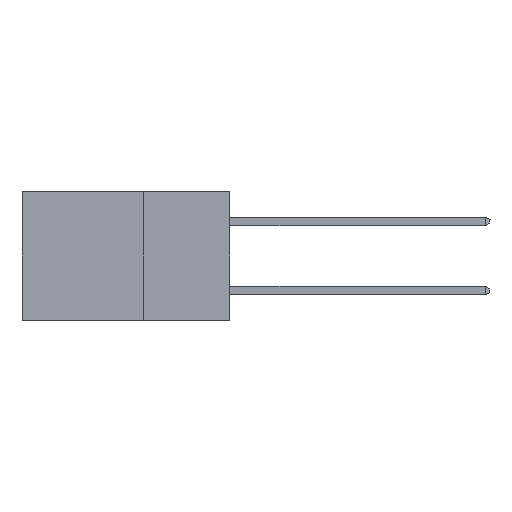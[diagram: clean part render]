
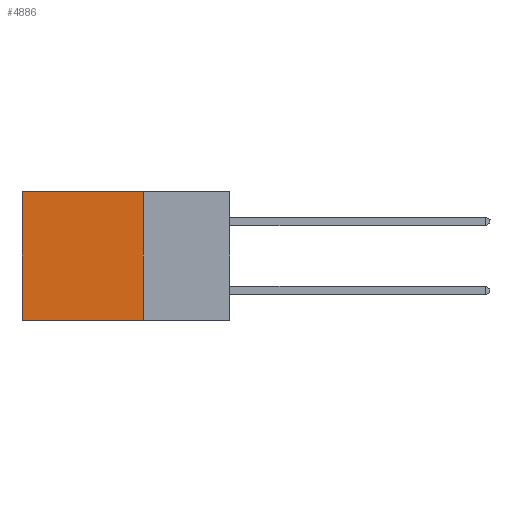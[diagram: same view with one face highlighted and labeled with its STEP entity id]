
A CAD part, left-side view. The second image highlights one B-rep face of the part: STEP entity #4886.
In plain terms, the highlighted planar face has unit normal (-1, 0, 0).
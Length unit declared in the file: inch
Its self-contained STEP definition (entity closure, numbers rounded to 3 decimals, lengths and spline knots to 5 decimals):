
#409 = LINE ( 'NONE', #14651, #15612 ) ;
#1426 = CARTESIAN_POINT ( 'NONE',  ( 0.298, 0.25, 0. ) ) ;
#1566 = CARTESIAN_POINT ( 'NONE',  ( 0.298, 0.6, 0. ) ) ;
#1586 = CARTESIAN_POINT ( 'NONE',  ( 0.298, 0.25, 0. ) ) ;
#1851 = VERTEX_POINT ( 'NONE', #18254 ) ;
#2798 = VERTEX_POINT ( 'NONE', #16984 ) ;
#3162 = DIRECTION ( 'NONE',  ( 0., 0., -1. ) ) ;
#4151 = ORIENTED_EDGE ( 'NONE', *, *, #17214, .F. ) ;
#4886 = ADVANCED_FACE ( 'NONE', ( #16403 ), #5881, .F. ) ;
#5252 = DIRECTION ( 'NONE',  ( 0., 0., -1. ) ) ;
#5590 = DIRECTION ( 'NONE',  ( 1., 0., 0. ) ) ;
#5627 = EDGE_LOOP ( 'NONE', ( #13952, #15307, #4151, #10874 ) ) ;
#5881 = PLANE ( 'NONE',  #12625 ) ;
#5954 = LINE ( 'NONE', #1426, #8982 ) ;
#6036 = CARTESIAN_POINT ( 'NONE',  ( 0.298, 0.25, 0. ) ) ;
#8509 = VERTEX_POINT ( 'NONE', #13135 ) ;
#8934 = DIRECTION ( 'NONE',  ( 0., 0., -1. ) ) ;
#8982 = VECTOR ( 'NONE', #8934, 39.37008 ) ;
#9038 = VECTOR ( 'NONE', #3162, 39.37008 ) ;
#9084 = DIRECTION ( 'NONE',  ( 0., 1., 0. ) ) ;
#10016 = DIRECTION ( 'NONE',  ( 0., 1., 0. ) ) ;
#10062 = CARTESIAN_POINT ( 'NONE',  ( 0.298, 0.25, 0. ) ) ;
#10158 = VECTOR ( 'NONE', #9084, 39.37008 ) ;
#10874 = ORIENTED_EDGE ( 'NONE', *, *, #12608, .T. ) ;
#12357 = VERTEX_POINT ( 'NONE', #10062 ) ;
#12608 = EDGE_CURVE ( 'NONE', #12357, #8509, #13285, .T. ) ;
#12625 = AXIS2_PLACEMENT_3D ( 'NONE', #6036, #5590, #5252 ) ;
#13135 = CARTESIAN_POINT ( 'NONE',  ( 0.298, 0.6, 0. ) ) ;
#13285 = LINE ( 'NONE', #1586, #10158 ) ;
#13952 = ORIENTED_EDGE ( 'NONE', *, *, #19276, .T. ) ;
#14651 = CARTESIAN_POINT ( 'NONE',  ( 0.298, 0.25, -0.37 ) ) ;
#15307 = ORIENTED_EDGE ( 'NONE', *, *, #17686, .F. ) ;
#15612 = VECTOR ( 'NONE', #10016, 39.37008 ) ;
#16403 = FACE_OUTER_BOUND ( 'NONE', #5627, .T. ) ;
#16984 = CARTESIAN_POINT ( 'NONE',  ( 0.298, 0.25, -0.37 ) ) ;
#17054 = LINE ( 'NONE', #1566, #9038 ) ;
#17214 = EDGE_CURVE ( 'NONE', #12357, #2798, #5954, .T. ) ;
#17686 = EDGE_CURVE ( 'NONE', #2798, #1851, #409, .T. ) ;
#18254 = CARTESIAN_POINT ( 'NONE',  ( 0.298, 0.6, -0.37 ) ) ;
#19276 = EDGE_CURVE ( 'NONE', #8509, #1851, #17054, .T. ) ;
